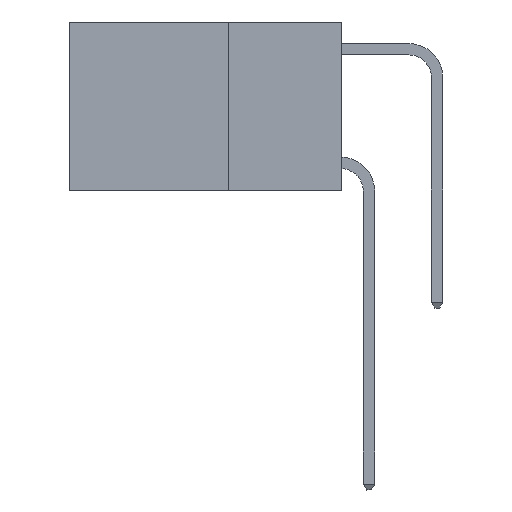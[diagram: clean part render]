
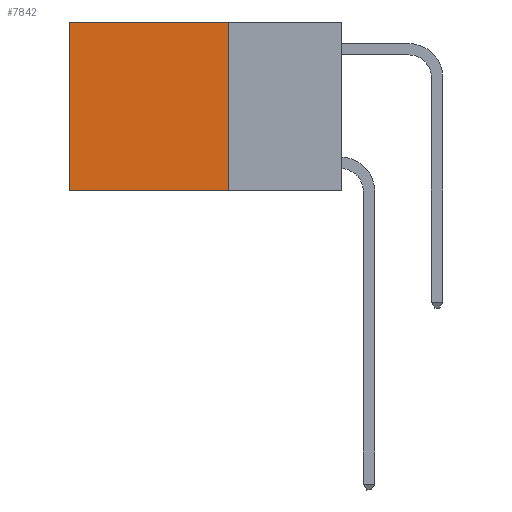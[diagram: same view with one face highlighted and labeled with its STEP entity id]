
A CAD part, left-side view. The second image highlights one B-rep face of the part: STEP entity #7842.
In plain terms, the highlighted planar face has unit normal (-1, 0, 0).
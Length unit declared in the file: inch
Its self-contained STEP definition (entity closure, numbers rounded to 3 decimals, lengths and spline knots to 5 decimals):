
#1814 = CARTESIAN_POINT ( 'NONE',  ( 0.2625, 0.6, 0. ) ) ;
#4102 = DIRECTION ( 'NONE',  ( 0., 1., 0. ) ) ;
#4352 = VECTOR ( 'NONE', #6885, 39.37008 ) ;
#6597 = DIRECTION ( 'NONE',  ( 1., 0., 0. ) ) ;
#6885 = DIRECTION ( 'NONE',  ( 0., 0., -1. ) ) ;
#7059 = EDGE_LOOP ( 'NONE', ( #13378, #8888, #19351, #22758 ) ) ;
#7173 = EDGE_CURVE ( 'NONE', #7256, #26168, #19154, .T. ) ;
#7256 = VERTEX_POINT ( 'NONE', #25487 ) ;
#7842 = ADVANCED_FACE ( 'NONE', ( #16097 ), #21632, .F. ) ;
#8271 = CARTESIAN_POINT ( 'NONE',  ( 0.2625, 0.6, -0.37 ) ) ;
#8502 = CARTESIAN_POINT ( 'NONE',  ( 0.2625, 0.25, 0. ) ) ;
#8888 = ORIENTED_EDGE ( 'NONE', *, *, #18988, .F. ) ;
#9820 = VECTOR ( 'NONE', #27274, 39.37008 ) ;
#10101 = EDGE_CURVE ( 'NONE', #7256, #16258, #16028, .T. ) ;
#10137 = AXIS2_PLACEMENT_3D ( 'NONE', #18870, #6597, #31415 ) ;
#10606 = LINE ( 'NONE', #20417, #16551 ) ;
#10856 = CARTESIAN_POINT ( 'NONE',  ( 0.2625, 0.25, -0.37 ) ) ;
#12242 = EDGE_CURVE ( 'NONE', #16258, #31320, #32185, .T. ) ;
#13378 = ORIENTED_EDGE ( 'NONE', *, *, #12242, .T. ) ;
#14403 = CARTESIAN_POINT ( 'NONE',  ( 0.2625, 0.25, 0. ) ) ;
#16028 = LINE ( 'NONE', #8502, #29537 ) ;
#16097 = FACE_OUTER_BOUND ( 'NONE', #7059, .T. ) ;
#16258 = VERTEX_POINT ( 'NONE', #22489 ) ;
#16551 = VECTOR ( 'NONE', #20736, 39.37008 ) ;
#18870 = CARTESIAN_POINT ( 'NONE',  ( 0.2625, 0.25, 0. ) ) ;
#18988 = EDGE_CURVE ( 'NONE', #26168, #31320, #10606, .T. ) ;
#19154 = LINE ( 'NONE', #14403, #4352 ) ;
#19351 = ORIENTED_EDGE ( 'NONE', *, *, #7173, .F. ) ;
#20417 = CARTESIAN_POINT ( 'NONE',  ( 0.2625, 0.25, -0.37 ) ) ;
#20736 = DIRECTION ( 'NONE',  ( 0., 1., 0. ) ) ;
#21632 = PLANE ( 'NONE',  #10137 ) ;
#22489 = CARTESIAN_POINT ( 'NONE',  ( 0.2625, 0.6, 0. ) ) ;
#22758 = ORIENTED_EDGE ( 'NONE', *, *, #10101, .T. ) ;
#25487 = CARTESIAN_POINT ( 'NONE',  ( 0.2625, 0.25, 0. ) ) ;
#26168 = VERTEX_POINT ( 'NONE', #10856 ) ;
#27274 = DIRECTION ( 'NONE',  ( 0., 0., -1. ) ) ;
#29537 = VECTOR ( 'NONE', #4102, 39.37008 ) ;
#31320 = VERTEX_POINT ( 'NONE', #8271 ) ;
#31415 = DIRECTION ( 'NONE',  ( 0., 0., -1. ) ) ;
#32185 = LINE ( 'NONE', #1814, #9820 ) ;
